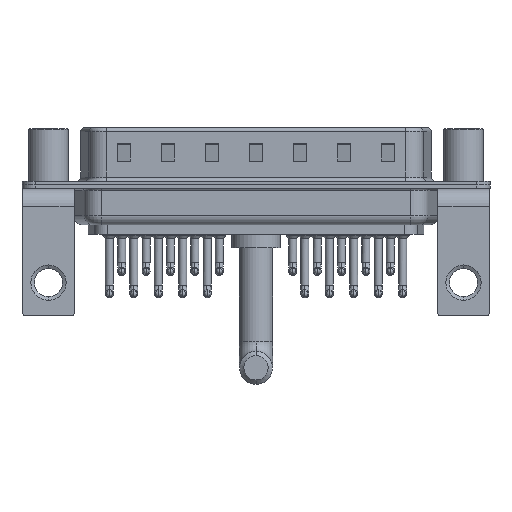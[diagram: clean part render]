
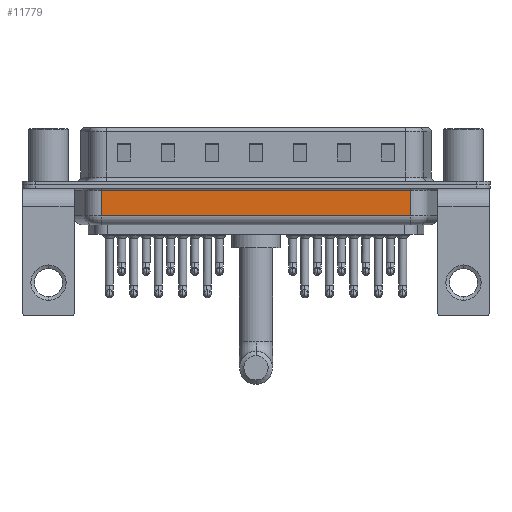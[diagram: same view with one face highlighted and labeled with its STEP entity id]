
A CAD part, front view. The second image highlights one B-rep face of the part: STEP entity #11779.
In plain terms, the highlighted planar face has unit normal (0, -1, 0).
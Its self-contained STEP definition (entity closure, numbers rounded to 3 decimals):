
#243 = CARTESIAN_POINT ( 'NONE',  ( 41.044, -5.35, -0.65 ) ) ;
#259 = CARTESIAN_POINT ( 'NONE',  ( 6.006, -5.35, -4.5 ) ) ;
#434 = LINE ( 'NONE', #4891, #26049 ) ;
#500 = ORIENTED_EDGE ( 'NONE', *, *, #19936, .T. ) ;
#534 = VERTEX_POINT ( 'NONE', #18414 ) ;
#1096 = ORIENTED_EDGE ( 'NONE', *, *, #5800, .T. ) ;
#1415 = CARTESIAN_POINT ( 'NONE',  ( 41.044, -5.35, -4.5 ) ) ;
#2370 = EDGE_CURVE ( 'NONE', #26347, #534, #15903, .T. ) ;
#4891 = CARTESIAN_POINT ( 'NONE',  ( 6.006, -5.35, -3.5 ) ) ;
#5602 = EDGE_LOOP ( 'NONE', ( #13512, #1096, #500, #22262 ) ) ;
#5800 = EDGE_CURVE ( 'NONE', #20526, #7017, #434, .T. ) ;
#7017 = VERTEX_POINT ( 'NONE', #8034 ) ;
#7576 = DIRECTION ( 'NONE',  ( -1., 0., 0. ) ) ;
#7885 = LINE ( 'NONE', #1415, #26724 ) ;
#8034 = CARTESIAN_POINT ( 'NONE',  ( 41.044, -5.35, -3.5 ) ) ;
#8446 = EDGE_CURVE ( 'NONE', #20526, #534, #8904, .T. ) ;
#8798 = CARTESIAN_POINT ( 'NONE',  ( 6.006, -5.35, -4.5 ) ) ;
#8904 = LINE ( 'NONE', #259, #14697 ) ;
#9082 = PLANE ( 'NONE',  #28135 ) ;
#10175 = DIRECTION ( 'NONE',  ( 0., 0., 1. ) ) ;
#11065 = DIRECTION ( 'NONE',  ( 1., 0., 0. ) ) ;
#11079 = DIRECTION ( 'NONE',  ( 0., 0., 1. ) ) ;
#11779 = ADVANCED_FACE ( 'NONE', ( #17982 ), #9082, .F. ) ;
#12952 = DIRECTION ( 'NONE',  ( 0., 1., 0. ) ) ;
#13512 = ORIENTED_EDGE ( 'NONE', *, *, #8446, .F. ) ;
#14697 = VECTOR ( 'NONE', #15495, 1000. ) ;
#15495 = DIRECTION ( 'NONE',  ( 0., 0., 1. ) ) ;
#15903 = LINE ( 'NONE', #27247, #25356 ) ;
#17982 = FACE_OUTER_BOUND ( 'NONE', #5602, .T. ) ;
#18414 = CARTESIAN_POINT ( 'NONE',  ( 6.006, -5.35, -0.65 ) ) ;
#19936 = EDGE_CURVE ( 'NONE', #7017, #26347, #7885, .T. ) ;
#20526 = VERTEX_POINT ( 'NONE', #24066 ) ;
#22262 = ORIENTED_EDGE ( 'NONE', *, *, #2370, .T. ) ;
#24066 = CARTESIAN_POINT ( 'NONE',  ( 6.006, -5.35, -3.5 ) ) ;
#25356 = VECTOR ( 'NONE', #7576, 1000. ) ;
#26049 = VECTOR ( 'NONE', #11065, 1000. ) ;
#26347 = VERTEX_POINT ( 'NONE', #243 ) ;
#26724 = VECTOR ( 'NONE', #10175, 1000. ) ;
#27247 = CARTESIAN_POINT ( 'NONE',  ( 6.006, -5.35, -0.65 ) ) ;
#28135 = AXIS2_PLACEMENT_3D ( 'NONE', #8798, #12952, #11079 ) ;
